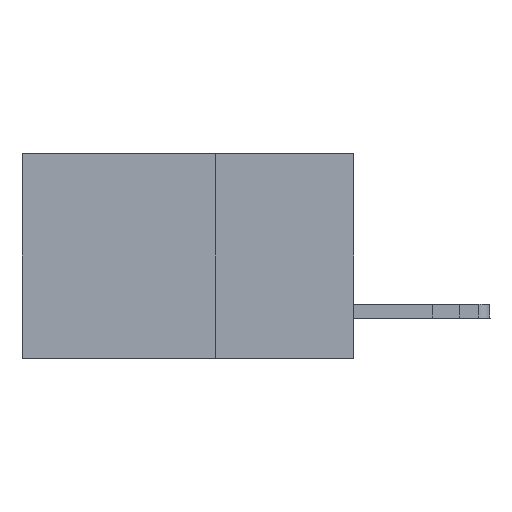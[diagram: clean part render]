
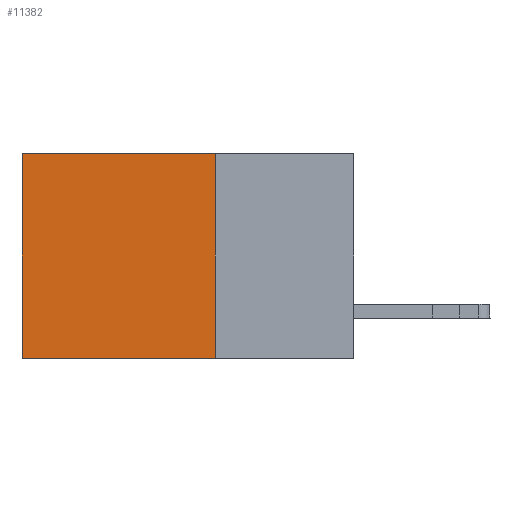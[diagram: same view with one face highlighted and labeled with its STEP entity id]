
A CAD part, left-side view. The second image highlights one B-rep face of the part: STEP entity #11382.
In plain terms, the highlighted planar face has unit normal (-1, 0, 0).
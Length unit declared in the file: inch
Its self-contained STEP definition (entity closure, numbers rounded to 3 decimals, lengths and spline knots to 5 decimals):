
#963 = CARTESIAN_POINT ( 'NONE',  ( 0.2875, 0.25, 0. ) ) ;
#2632 = PLANE ( 'NONE',  #22921 ) ;
#3698 = LINE ( 'NONE', #963, #16182 ) ;
#4548 = CARTESIAN_POINT ( 'NONE',  ( 0.2875, 0.25, -0.37 ) ) ;
#4627 = VECTOR ( 'NONE', #12076, 39.37008 ) ;
#6247 = CARTESIAN_POINT ( 'NONE',  ( 0.2875, 0.25, 0. ) ) ;
#6898 = VERTEX_POINT ( 'NONE', #12808 ) ;
#10144 = DIRECTION ( 'NONE',  ( 1., 0., 0. ) ) ;
#10187 = FACE_OUTER_BOUND ( 'NONE', #15183, .T. ) ;
#10372 = VECTOR ( 'NONE', #30197, 39.37008 ) ;
#10933 = CARTESIAN_POINT ( 'NONE',  ( 0.2875, 0.6, 0. ) ) ;
#11112 = EDGE_CURVE ( 'NONE', #24526, #19382, #31149, .T. ) ;
#11267 = LINE ( 'NONE', #4548, #4627 ) ;
#11382 = ADVANCED_FACE ( 'NONE', ( #10187 ), #2632, .F. ) ;
#12076 = DIRECTION ( 'NONE',  ( 0., 1., 0. ) ) ;
#12161 = VECTOR ( 'NONE', #23605, 39.37008 ) ;
#12808 = CARTESIAN_POINT ( 'NONE',  ( 0.2875, 0.25, -0.37 ) ) ;
#13602 = ORIENTED_EDGE ( 'NONE', *, *, #21823, .F. ) ;
#15183 = EDGE_LOOP ( 'NONE', ( #31901, #13602, #19695, #22418 ) ) ;
#16182 = VECTOR ( 'NONE', #23322, 39.37008 ) ;
#17006 = LINE ( 'NONE', #22727, #10372 ) ;
#19382 = VERTEX_POINT ( 'NONE', #10933 ) ;
#19695 = ORIENTED_EDGE ( 'NONE', *, *, #24061, .F. ) ;
#20902 = CARTESIAN_POINT ( 'NONE',  ( 0.2875, 0.6, -0.37 ) ) ;
#21823 = EDGE_CURVE ( 'NONE', #6898, #27791, #11267, .T. ) ;
#22418 = ORIENTED_EDGE ( 'NONE', *, *, #11112, .T. ) ;
#22508 = CARTESIAN_POINT ( 'NONE',  ( 0.2875, 0.25, 0. ) ) ;
#22727 = CARTESIAN_POINT ( 'NONE',  ( 0.2875, 0.6, 0. ) ) ;
#22921 = AXIS2_PLACEMENT_3D ( 'NONE', #25021, #10144, #27525 ) ;
#23322 = DIRECTION ( 'NONE',  ( 0., 0., -1. ) ) ;
#23605 = DIRECTION ( 'NONE',  ( 0., 1., 0. ) ) ;
#24061 = EDGE_CURVE ( 'NONE', #24526, #6898, #3698, .T. ) ;
#24526 = VERTEX_POINT ( 'NONE', #22508 ) ;
#25021 = CARTESIAN_POINT ( 'NONE',  ( 0.2875, 0.25, 0. ) ) ;
#26452 = EDGE_CURVE ( 'NONE', #19382, #27791, #17006, .T. ) ;
#27525 = DIRECTION ( 'NONE',  ( 0., 0., -1. ) ) ;
#27791 = VERTEX_POINT ( 'NONE', #20902 ) ;
#30197 = DIRECTION ( 'NONE',  ( 0., 0., -1. ) ) ;
#31149 = LINE ( 'NONE', #6247, #12161 ) ;
#31901 = ORIENTED_EDGE ( 'NONE', *, *, #26452, .T. ) ;
